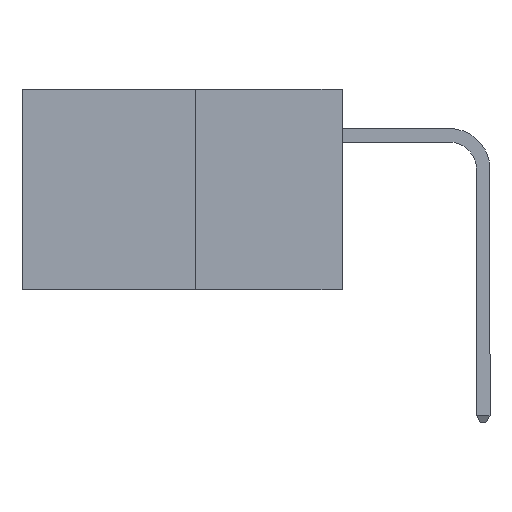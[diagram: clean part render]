
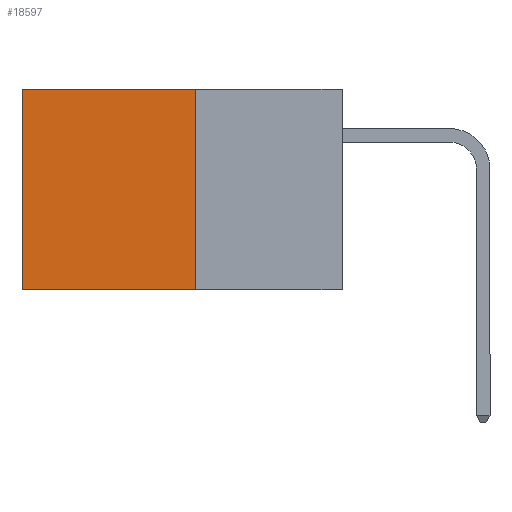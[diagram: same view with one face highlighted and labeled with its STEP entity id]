
A CAD part, left-side view. The second image highlights one B-rep face of the part: STEP entity #18597.
In plain terms, the highlighted planar face has unit normal (-1, 0, 0).
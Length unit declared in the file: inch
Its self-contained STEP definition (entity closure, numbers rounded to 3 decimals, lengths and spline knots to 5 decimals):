
#354 = DIRECTION ( 'NONE',  ( 0., 0., -1. ) ) ;
#1373 = DIRECTION ( 'NONE',  ( 0., 1., 0. ) ) ;
#2888 = ORIENTED_EDGE ( 'NONE', *, *, #28519, .F. ) ;
#3188 = CARTESIAN_POINT ( 'NONE',  ( 0.277, 0.59, -0.37 ) ) ;
#3500 = LINE ( 'NONE', #23890, #15682 ) ;
#4846 = VERTEX_POINT ( 'NONE', #3188 ) ;
#5548 = VECTOR ( 'NONE', #1373, 39.37008 ) ;
#5975 = ORIENTED_EDGE ( 'NONE', *, *, #13118, .T. ) ;
#6817 = PLANE ( 'NONE',  #20690 ) ;
#7150 = EDGE_CURVE ( 'NONE', #10574, #4846, #20064, .T. ) ;
#10137 = VERTEX_POINT ( 'NONE', #25044 ) ;
#10574 = VERTEX_POINT ( 'NONE', #31509 ) ;
#11716 = DIRECTION ( 'NONE',  ( 1., 0., 0. ) ) ;
#11755 = LINE ( 'NONE', #23771, #23985 ) ;
#12791 = LINE ( 'NONE', #16019, #5548 ) ;
#13118 = EDGE_CURVE ( 'NONE', #10137, #10574, #12791, .T. ) ;
#15006 = CARTESIAN_POINT ( 'NONE',  ( 0.277, 0.59, -0.37 ) ) ;
#15472 = EDGE_LOOP ( 'NONE', ( #21478, #2888, #16943, #5975 ) ) ;
#15682 = VECTOR ( 'NONE', #21435, 39.37008 ) ;
#16019 = CARTESIAN_POINT ( 'NONE',  ( 0.277, 0.27, 0. ) ) ;
#16609 = DIRECTION ( 'NONE',  ( 0., 0., -1. ) ) ;
#16943 = ORIENTED_EDGE ( 'NONE', *, *, #26120, .F. ) ;
#17276 = CARTESIAN_POINT ( 'NONE',  ( 0.277, 0.27, -0.37 ) ) ;
#18597 = ADVANCED_FACE ( 'NONE', ( #19469 ), #6817, .F. ) ;
#19469 = FACE_OUTER_BOUND ( 'NONE', #15472, .T. ) ;
#20064 = LINE ( 'NONE', #15006, #27262 ) ;
#20690 = AXIS2_PLACEMENT_3D ( 'NONE', #23892, #11716, #28767 ) ;
#21435 = DIRECTION ( 'NONE',  ( 0., 1., 0. ) ) ;
#21478 = ORIENTED_EDGE ( 'NONE', *, *, #7150, .T. ) ;
#21846 = VERTEX_POINT ( 'NONE', #17276 ) ;
#23771 = CARTESIAN_POINT ( 'NONE',  ( 0.277, 0.27, -0.37 ) ) ;
#23890 = CARTESIAN_POINT ( 'NONE',  ( 0.277, 0.27, -0.37 ) ) ;
#23892 = CARTESIAN_POINT ( 'NONE',  ( 0.277, 0.27, -0.37 ) ) ;
#23985 = VECTOR ( 'NONE', #16609, 39.37008 ) ;
#25044 = CARTESIAN_POINT ( 'NONE',  ( 0.277, 0.27, 0. ) ) ;
#26120 = EDGE_CURVE ( 'NONE', #10137, #21846, #11755, .T. ) ;
#27262 = VECTOR ( 'NONE', #354, 39.37008 ) ;
#28519 = EDGE_CURVE ( 'NONE', #21846, #4846, #3500, .T. ) ;
#28767 = DIRECTION ( 'NONE',  ( 0., 0., -1. ) ) ;
#31509 = CARTESIAN_POINT ( 'NONE',  ( 0.277, 0.59, 0. ) ) ;
